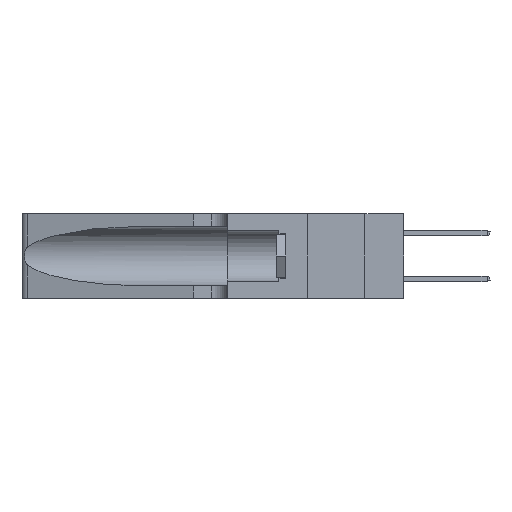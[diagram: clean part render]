
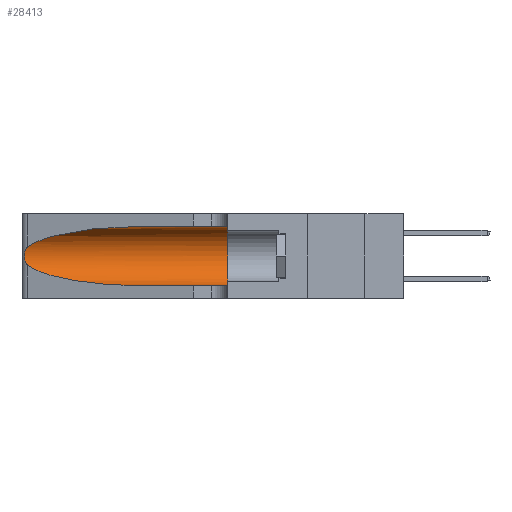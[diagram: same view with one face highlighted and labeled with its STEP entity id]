
A CAD part, left-side view. The second image highlights one B-rep face of the part: STEP entity #28413.
In plain terms, the highlighted cylindrical face has radius 3.308 mm (diameter 6.617 mm), a partial arc.
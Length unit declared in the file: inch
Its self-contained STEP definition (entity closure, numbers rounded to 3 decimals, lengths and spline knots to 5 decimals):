
#377 = CARTESIAN_POINT ( 'NONE',  ( 0.1305, 0.72297, 0.31525 ) ) ;
#453 = CARTESIAN_POINT ( 'NONE',  ( 0.1305, 0.72297, 0.31525 ) ) ;
#1698 = CARTESIAN_POINT ( 'NONE',  ( 0.1305, 0.72297, 0.05475 ) ) ;
#1838 = VERTEX_POINT ( 'NONE', #1986 ) ;
#1986 = CARTESIAN_POINT ( 'NONE',  ( 0.1305, 0.35, 0.31525 ) ) ;
#2588 = DIRECTION ( 'NONE',  ( 0., -1., 0. ) ) ;
#2686 =( BOUNDED_CURVE ( )  B_SPLINE_CURVE ( 3, ( #377, #12095, #5059, #27993 ),
 .UNSPECIFIED., .F., .F. ) 
 B_SPLINE_CURVE_WITH_KNOTS ( ( 4, 4 ),
 ( 1.5708, 2.84003 ),
 .UNSPECIFIED. ) 
 CURVE ( )  GEOMETRIC_REPRESENTATION_ITEM ( )  RATIONAL_B_SPLINE_CURVE ( ( 1., 0.87, 0.87, 1. ) ) 
 REPRESENTATION_ITEM ( '' )  );
#3305 = AXIS2_PLACEMENT_3D ( 'NONE', #9080, #20202, #15753 ) ;
#3329 = CYLINDRICAL_SURFACE ( 'NONE', #7816, 0.13025 ) ;
#3587 = ORIENTED_EDGE ( 'NONE', *, *, #23443, .T. ) ;
#3987 = VECTOR ( 'NONE', #2588, 39.37008 ) ;
#4750 = EDGE_CURVE ( 'NONE', #21019, #16192, #2686, .T. ) ;
#5059 = CARTESIAN_POINT ( 'NONE',  ( 0.2373, 1.15595, 0.28018 ) ) ;
#5062 = CARTESIAN_POINT ( 'NONE',  ( 0.1305, 1.61858, 0.05475 ) ) ;
#6694 = EDGE_CURVE ( 'NONE', #16192, #22786, #28728, .T. ) ;
#7694 = CIRCLE ( 'NONE', #3305, 0.13025 ) ;
#7816 = AXIS2_PLACEMENT_3D ( 'NONE', #29066, #8355, #24486 ) ;
#8355 = DIRECTION ( 'NONE',  ( 0., -1., 0. ) ) ;
#8476 = LINE ( 'NONE', #24268, #19848 ) ;
#8547 = CARTESIAN_POINT ( 'NONE',  ( 0.25555, 1.22994, 0.2215 ) ) ;
#8630 = CARTESIAN_POINT ( 'NONE',  ( 0.25639, 1.23184, 0.21858 ) ) ;
#8824 = CARTESIAN_POINT ( 'NONE',  ( 0.25787, 1.23484, 0.2124 ) ) ;
#8916 = CARTESIAN_POINT ( 'NONE',  ( 0.1305, 0.35, 0.05475 ) ) ;
#9080 = CARTESIAN_POINT ( 'NONE',  ( 0.1305, 0.35, 0.185 ) ) ;
#10412 = CARTESIAN_POINT ( 'NONE',  ( 0.2373, 1.15595, 0.08982 ) ) ;
#10517 = CARTESIAN_POINT ( 'NONE',  ( 0.18966, 0.96281, 0.05475 ) ) ;
#10645 = DIRECTION ( 'NONE',  ( 0., -1., 0. ) ) ;
#10763 = ORIENTED_EDGE ( 'NONE', *, *, #16455, .F. ) ;
#10932 = CARTESIAN_POINT ( 'NONE',  ( 0.26017, 1.23833, 0.17102 ) ) ;
#11129 = CARTESIAN_POINT ( 'NONE',  ( 0.25555, 1.22993, 0.14849 ) ) ;
#11734 = CARTESIAN_POINT ( 'NONE',  ( 0.25487, 1.22718, 0.14631 ) ) ;
#12095 = CARTESIAN_POINT ( 'NONE',  ( 0.18966, 0.96281, 0.31525 ) ) ;
#12557 = EDGE_CURVE ( 'NONE', #1838, #25517, #7694, .T. ) ;
#14369 = CARTESIAN_POINT ( 'NONE',  ( 0.25487, 1.22718, 0.22369 ) ) ;
#15381 = FACE_OUTER_BOUND ( 'NONE', #23468, .T. ) ;
#15496 = CARTESIAN_POINT ( 'NONE',  ( 0.25856, 1.23593, 0.16098 ) ) ;
#15753 = DIRECTION ( 'NONE',  ( 0., 0., 1. ) ) ;
#16192 = VERTEX_POINT ( 'NONE', #14369 ) ;
#16308 =( BOUNDED_CURVE ( )  B_SPLINE_CURVE ( 3, ( #24241, #10412, #10517, #1698 ),
 .UNSPECIFIED., .F., .T. ) 
 B_SPLINE_CURVE_WITH_KNOTS ( ( 4, 4 ),
 ( 3.44316, 4.71239 ),
 .UNSPECIFIED. ) 
 CURVE ( )  GEOMETRIC_REPRESENTATION_ITEM ( )  RATIONAL_B_SPLINE_CURVE ( ( 1., 0.87, 0.87, 1. ) ) 
 REPRESENTATION_ITEM ( '' )  );
#16455 = EDGE_CURVE ( 'NONE', #21019, #1838, #8476, .T. ) ;
#17775 = CARTESIAN_POINT ( 'NONE',  ( 0.26075, 1.23896, 0.178 ) ) ;
#19763 = CARTESIAN_POINT ( 'NONE',  ( 0.25854, 1.2359, 0.20912 ) ) ;
#19848 = VECTOR ( 'NONE', #10645, 39.37008 ) ;
#20202 = DIRECTION ( 'NONE',  ( 0., 1., 0. ) ) ;
#20780 = ORIENTED_EDGE ( 'NONE', *, *, #12557, .F. ) ;
#21019 = VERTEX_POINT ( 'NONE', #453 ) ;
#21734 = LINE ( 'NONE', #5062, #3987 ) ;
#22476 = CARTESIAN_POINT ( 'NONE',  ( 0.25487, 1.22718, 0.22369 ) ) ;
#22786 = VERTEX_POINT ( 'NONE', #11734 ) ;
#23443 = EDGE_CURVE ( 'NONE', #25242, #25517, #21734, .T. ) ;
#23468 = EDGE_LOOP ( 'NONE', ( #25990, #23859, #26118, #3587, #20780, #10763 ) ) ;
#23859 = ORIENTED_EDGE ( 'NONE', *, *, #6694, .T. ) ;
#24144 = CARTESIAN_POINT ( 'NONE',  ( 0.1305, 0.72297, 0.05475 ) ) ;
#24241 = CARTESIAN_POINT ( 'NONE',  ( 0.25487, 1.22718, 0.14631 ) ) ;
#24268 = CARTESIAN_POINT ( 'NONE',  ( 0.1305, 1.61858, 0.31525 ) ) ;
#24463 = CARTESIAN_POINT ( 'NONE',  ( 0.25789, 1.23486, 0.15765 ) ) ;
#24486 = DIRECTION ( 'NONE',  ( 0., 0., -1. ) ) ;
#24565 = CARTESIAN_POINT ( 'NONE',  ( 0.26018, 1.23835, 0.19895 ) ) ;
#24748 = CARTESIAN_POINT ( 'NONE',  ( 0.25639, 1.23186, 0.15144 ) ) ;
#25242 = VERTEX_POINT ( 'NONE', #24144 ) ;
#25517 = VERTEX_POINT ( 'NONE', #8916 ) ;
#25990 = ORIENTED_EDGE ( 'NONE', *, *, #4750, .T. ) ;
#26118 = ORIENTED_EDGE ( 'NONE', *, *, #28954, .T. ) ;
#27032 = CARTESIAN_POINT ( 'NONE',  ( 0.25487, 1.22718, 0.14631 ) ) ;
#27993 = CARTESIAN_POINT ( 'NONE',  ( 0.25487, 1.22718, 0.22369 ) ) ;
#28413 = ADVANCED_FACE ( 'NONE', ( #15381 ), #3329, .F. ) ;
#28728 = B_SPLINE_CURVE_WITH_KNOTS ( 'NONE', 3,
 ( #22476, #8547, #8630, #8824, #19763, #24565, #29139, #17775, #10932, #15496, #24463, #24748, #11129, #27032 ),
 .UNSPECIFIED., .F., .F.,
 ( 4, 2, 2, 2, 2, 2, 4 ),
 ( 0., 0.00027, 0.00053, 0.00107, 0.0016, 0.00187, 0.00214 ),
 .UNSPECIFIED. ) ;
#28954 = EDGE_CURVE ( 'NONE', #22786, #25242, #16308, .T. ) ;
#29066 = CARTESIAN_POINT ( 'NONE',  ( 0.1305, 1.61858, 0.185 ) ) ;
#29139 = CARTESIAN_POINT ( 'NONE',  ( 0.26075, 1.23896, 0.19203 ) ) ;
